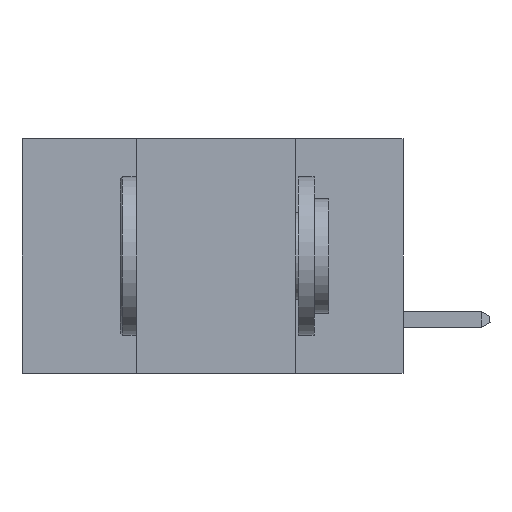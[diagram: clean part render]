
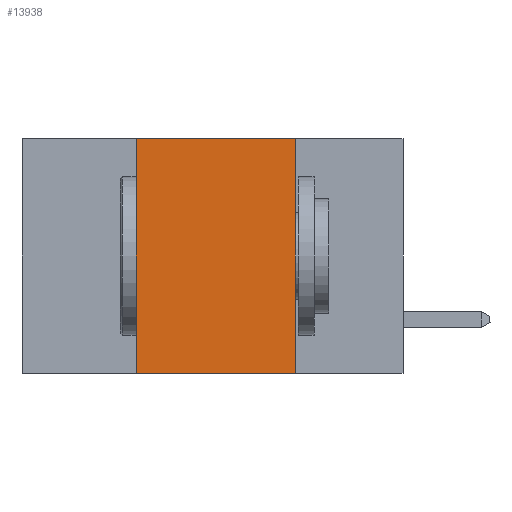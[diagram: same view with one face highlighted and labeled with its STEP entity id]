
A CAD part, left-side view. The second image highlights one B-rep face of the part: STEP entity #13938.
In plain terms, the highlighted planar face has unit normal (-1, 0, 0).
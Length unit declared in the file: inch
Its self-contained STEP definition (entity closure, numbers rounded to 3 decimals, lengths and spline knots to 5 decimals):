
#203 = VECTOR ( 'NONE', #12292, 39.37008 ) ;
#1117 = DIRECTION ( 'NONE',  ( 1., 0., 0. ) ) ;
#4210 = DIRECTION ( 'NONE',  ( 0., 0., -1. ) ) ;
#5199 = CARTESIAN_POINT ( 'NONE',  ( 0., 0.6, -0.37 ) ) ;
#5771 = LINE ( 'NONE', #41778, #13520 ) ;
#5809 = LINE ( 'NONE', #17298, #22427 ) ;
#6587 = CARTESIAN_POINT ( 'NONE',  ( 0., 0.42, -0.37 ) ) ;
#7128 = DIRECTION ( 'NONE',  ( 0., -1., 0. ) ) ;
#7523 = CARTESIAN_POINT ( 'NONE',  ( 0., 0.6, 0. ) ) ;
#8890 = VERTEX_POINT ( 'NONE', #6587 ) ;
#9565 = LINE ( 'NONE', #5199, #203 ) ;
#11272 = EDGE_LOOP ( 'NONE', ( #18156, #21889, #37248, #13194 ) ) ;
#11344 = CARTESIAN_POINT ( 'NONE',  ( 0., 0.17, -0.37 ) ) ;
#12292 = DIRECTION ( 'NONE',  ( 0., -1., 0. ) ) ;
#13194 = ORIENTED_EDGE ( 'NONE', *, *, #19565, .T. ) ;
#13520 = VECTOR ( 'NONE', #18707, 39.37008 ) ;
#13938 = ADVANCED_FACE ( 'NONE', ( #14160 ), #40176, .F. ) ;
#14160 = FACE_OUTER_BOUND ( 'NONE', #11272, .T. ) ;
#14456 = CARTESIAN_POINT ( 'NONE',  ( 0., 0.17, 0. ) ) ;
#16452 = CARTESIAN_POINT ( 'NONE',  ( 0., 0.42, 0. ) ) ;
#16572 = VERTEX_POINT ( 'NONE', #40850 ) ;
#17223 = VERTEX_POINT ( 'NONE', #11344 ) ;
#17298 = CARTESIAN_POINT ( 'NONE',  ( 0., 0.6, 0. ) ) ;
#18156 = ORIENTED_EDGE ( 'NONE', *, *, #41952, .F. ) ;
#18707 = DIRECTION ( 'NONE',  ( 0., 0., 1. ) ) ;
#19565 = EDGE_CURVE ( 'NONE', #8890, #17223, #9565, .T. ) ;
#21123 = EDGE_CURVE ( 'NONE', #40976, #16572, #5809, .T. ) ;
#21163 = LINE ( 'NONE', #14456, #33526 ) ;
#21409 = EDGE_CURVE ( 'NONE', #8890, #40976, #5771, .T. ) ;
#21889 = ORIENTED_EDGE ( 'NONE', *, *, #21123, .F. ) ;
#22427 = VECTOR ( 'NONE', #7128, 39.37008 ) ;
#31120 = DIRECTION ( 'NONE',  ( 0., 0., -1. ) ) ;
#33526 = VECTOR ( 'NONE', #31120, 39.37008 ) ;
#37248 = ORIENTED_EDGE ( 'NONE', *, *, #21409, .F. ) ;
#38349 = AXIS2_PLACEMENT_3D ( 'NONE', #7523, #1117, #4210 ) ;
#40176 = PLANE ( 'NONE',  #38349 ) ;
#40850 = CARTESIAN_POINT ( 'NONE',  ( 0., 0.17, 0. ) ) ;
#40976 = VERTEX_POINT ( 'NONE', #16452 ) ;
#41778 = CARTESIAN_POINT ( 'NONE',  ( 0., 0.42, 0. ) ) ;
#41952 = EDGE_CURVE ( 'NONE', #16572, #17223, #21163, .T. ) ;
